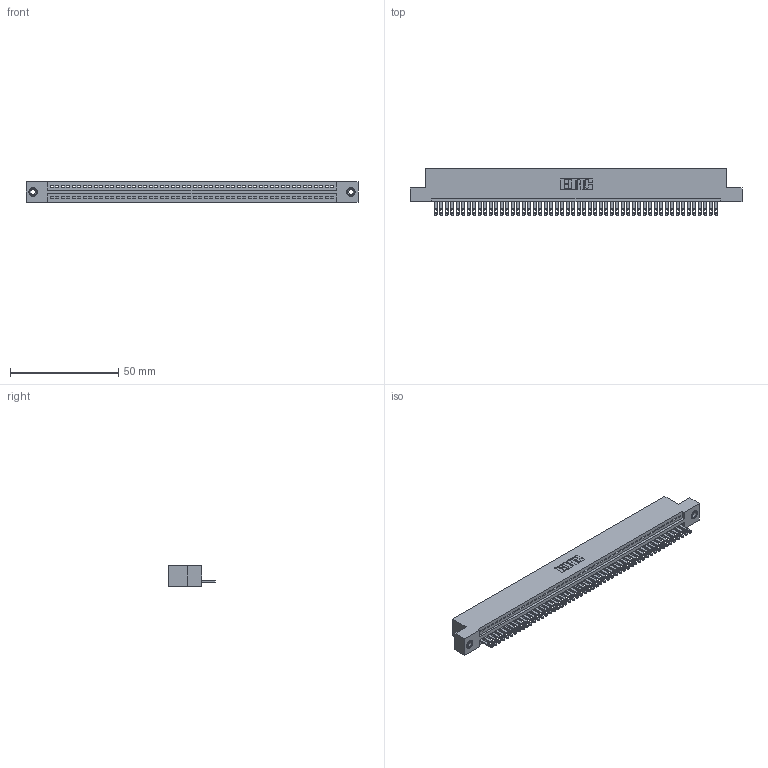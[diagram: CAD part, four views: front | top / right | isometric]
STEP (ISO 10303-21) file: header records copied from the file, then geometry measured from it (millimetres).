
FILE_DESCRIPTION (( 'STEP AP203' ), '1' );
FILE_NAME ('345-052-500-108.STEP', '2018-09-22T19:04:22', ( '' ), ( '' ), 'SwSTEP 2.0', 'SolidWorks 2016', '' );
FILE_SCHEMA (( 'CONFIG_CONTROL_DESIGN' ));
Length unit declared in the file: inch
Products named in the file (4): 345-292-001_345-293-100; 345-250-001_345-250-003-102; 345-052-500-108; 345 Part_Flush Mounting Lugs - 0.156 Dia-TI
Assembly tree (55 placements, depth 2):
  345-052-500-108
    345 Part_Flush Mounting Lugs - 0.156 Dia-TI
    345-292-001_345-293-100  x52
    345-250-001_345-250-003-102  x2
Bounding box: 153.29 x 21.51 x 9.4 mm (x, y, z)
Volume: 14667.1 mm3; surface area: 19763.1 mm2
Topology: 55 solids, 55 shells, 2994 faces, 9213 edges, 6134 vertices
Faces by surface type: plane 1880, cylinder 1098, cone 12, torus 4
Entity records: 38906 total; most frequent: CARTESIAN_POINT 6719, ORIENTED_EDGE 6698, DIRECTION 5883, EDGE_CURVE 3349, VECTOR 2985, LINE 2985, VERTEX_POINT 2228, AXIS2_PLACEMENT_3D 1449
